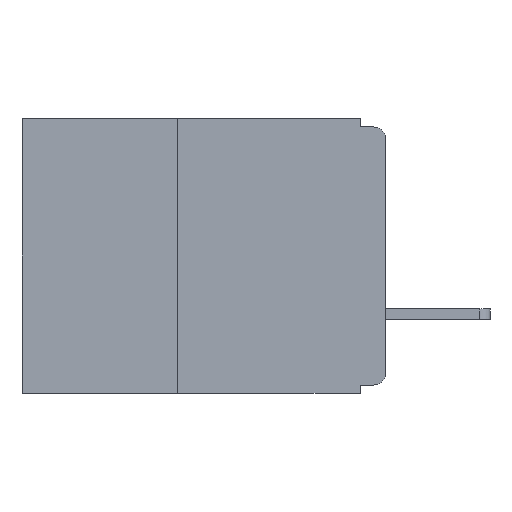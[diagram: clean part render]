
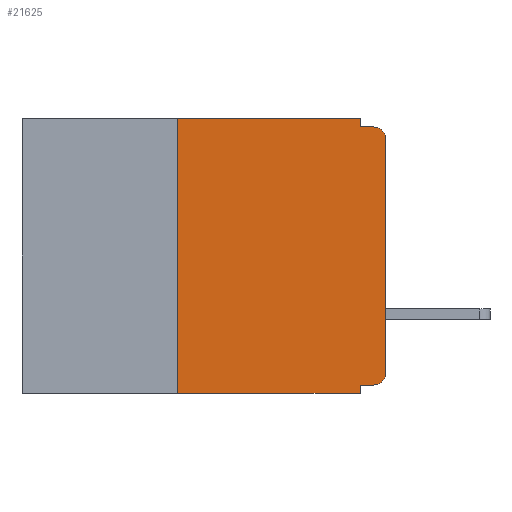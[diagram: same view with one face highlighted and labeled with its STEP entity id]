
A CAD part, left-side view. The second image highlights one B-rep face of the part: STEP entity #21625.
In plain terms, the highlighted planar face has unit normal (-1, 0, 0).
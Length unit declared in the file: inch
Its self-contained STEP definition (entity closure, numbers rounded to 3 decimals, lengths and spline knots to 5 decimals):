
#782 = DIRECTION ( 'NONE',  ( 0., -1., 0. ) ) ;
#1900 = ORIENTED_EDGE ( 'NONE', *, *, #23454, .F. ) ;
#1910 = VERTEX_POINT ( 'NONE', #27056 ) ;
#2072 = VECTOR ( 'NONE', #27822, 39.37008 ) ;
#3040 = CARTESIAN_POINT ( 'NONE',  ( 0., 0.031, -0.01 ) ) ;
#3853 = CARTESIAN_POINT ( 'NONE',  ( 0., 0.031, -0.33 ) ) ;
#4433 = VERTEX_POINT ( 'NONE', #3853 ) ;
#5592 = ORIENTED_EDGE ( 'NONE', *, *, #25178, .F. ) ;
#6671 = VERTEX_POINT ( 'NONE', #10846 ) ;
#6710 = EDGE_CURVE ( 'NONE', #1910, #20465, #29688, .T. ) ;
#7368 = LINE ( 'NONE', #30881, #26760 ) ;
#7585 = CARTESIAN_POINT ( 'NONE',  ( 0., 0.031, 0. ) ) ;
#7941 = CARTESIAN_POINT ( 'NONE',  ( 0., 0.25, -0.33 ) ) ;
#8379 = CIRCLE ( 'NONE', #24400, 0.015 ) ;
#8435 = ORIENTED_EDGE ( 'NONE', *, *, #30061, .T. ) ;
#8722 = VERTEX_POINT ( 'NONE', #14818 ) ;
#9685 = DIRECTION ( 'NONE',  ( 0., 0., -1. ) ) ;
#9710 = DIRECTION ( 'NONE',  ( -1., 0., 0. ) ) ;
#9717 = CARTESIAN_POINT ( 'NONE',  ( 0., 0.015, -0.025 ) ) ;
#9826 = DIRECTION ( 'NONE',  ( 0., 1., 0. ) ) ;
#9896 = AXIS2_PLACEMENT_3D ( 'NONE', #9717, #9710, #9685 ) ;
#10846 = CARTESIAN_POINT ( 'NONE',  ( 0., 0.031, 0. ) ) ;
#11538 = CARTESIAN_POINT ( 'NONE',  ( 0., 0.015, -0.305 ) ) ;
#11720 = VECTOR ( 'NONE', #9826, 39.37008 ) ;
#11738 = ORIENTED_EDGE ( 'NONE', *, *, #24427, .T. ) ;
#12065 = EDGE_CURVE ( 'NONE', #8722, #18976, #19317, .T. ) ;
#12128 = ORIENTED_EDGE ( 'NONE', *, *, #26253, .F. ) ;
#12326 = CARTESIAN_POINT ( 'NONE',  ( 0., 0.25, -0.33 ) ) ;
#13270 = FACE_OUTER_BOUND ( 'NONE', #25544, .T. ) ;
#13372 = DIRECTION ( 'NONE',  ( 1., 0., 0. ) ) ;
#13561 = DIRECTION ( 'NONE',  ( 0., -1., 0. ) ) ;
#13675 = VECTOR ( 'NONE', #21478, 39.37008 ) ;
#13900 = CARTESIAN_POINT ( 'NONE',  ( 0., 0.437, 0. ) ) ;
#14158 = DIRECTION ( 'NONE',  ( 0., 0., -1. ) ) ;
#14600 = ORIENTED_EDGE ( 'NONE', *, *, #25430, .F. ) ;
#14818 = CARTESIAN_POINT ( 'NONE',  ( 0., 0.015, -0.32 ) ) ;
#14859 = CARTESIAN_POINT ( 'NONE',  ( 0., 0., -0.32 ) ) ;
#15343 = CARTESIAN_POINT ( 'NONE',  ( 0., 0., -0.305 ) ) ;
#15831 = ORIENTED_EDGE ( 'NONE', *, *, #12065, .F. ) ;
#16250 = VECTOR ( 'NONE', #13561, 39.37008 ) ;
#16925 = ORIENTED_EDGE ( 'NONE', *, *, #6710, .T. ) ;
#17311 = VECTOR ( 'NONE', #32391, 39.37008 ) ;
#17807 = VERTEX_POINT ( 'NONE', #3040 ) ;
#18728 = VECTOR ( 'NONE', #27513, 39.37008 ) ;
#18751 = VERTEX_POINT ( 'NONE', #29865 ) ;
#18976 = VERTEX_POINT ( 'NONE', #26283 ) ;
#19317 = LINE ( 'NONE', #14859, #11720 ) ;
#20465 = VERTEX_POINT ( 'NONE', #27160 ) ;
#21439 = CARTESIAN_POINT ( 'NONE',  ( 0., 0., -0.01 ) ) ;
#21478 = DIRECTION ( 'NONE',  ( 0., -1., 0. ) ) ;
#21625 = ADVANCED_FACE ( 'NONE', ( #13270 ), #23345, .F. ) ;
#21923 = LINE ( 'NONE', #13900, #13675 ) ;
#22624 = EDGE_CURVE ( 'NONE', #6671, #17807, #29143, .T. ) ;
#23169 = ORIENTED_EDGE ( 'NONE', *, *, #22624, .F. ) ;
#23345 = PLANE ( 'NONE',  #32097 ) ;
#23454 = EDGE_CURVE ( 'NONE', #18976, #4433, #7368, .T. ) ;
#23763 = DIRECTION ( 'NONE',  ( 0., 0., -1. ) ) ;
#23917 = LINE ( 'NONE', #12326, #17311 ) ;
#24400 = AXIS2_PLACEMENT_3D ( 'NONE', #11538, #29065, #14158 ) ;
#24427 = EDGE_CURVE ( 'NONE', #26658, #4433, #29389, .T. ) ;
#24512 = LINE ( 'NONE', #25033, #18728 ) ;
#25033 = CARTESIAN_POINT ( 'NONE',  ( 0., 0., 0. ) ) ;
#25178 = EDGE_CURVE ( 'NONE', #17807, #20465, #25889, .T. ) ;
#25430 = EDGE_CURVE ( 'NONE', #26658, #18751, #23917, .T. ) ;
#25544 = EDGE_LOOP ( 'NONE', ( #8435, #16925, #5592, #23169, #12128, #14600, #11738, #1900, #15831, #32851 ) ) ;
#25889 = LINE ( 'NONE', #21439, #31648 ) ;
#26253 = EDGE_CURVE ( 'NONE', #18751, #6671, #21923, .T. ) ;
#26283 = CARTESIAN_POINT ( 'NONE',  ( 0., 0.031, -0.32 ) ) ;
#26658 = VERTEX_POINT ( 'NONE', #7941 ) ;
#26760 = VECTOR ( 'NONE', #23763, 39.37008 ) ;
#27056 = CARTESIAN_POINT ( 'NONE',  ( 0., 0., -0.025 ) ) ;
#27160 = CARTESIAN_POINT ( 'NONE',  ( 0., 0.015, -0.01 ) ) ;
#27513 = DIRECTION ( 'NONE',  ( 0., 0., 1. ) ) ;
#27822 = DIRECTION ( 'NONE',  ( 0., 0., -1. ) ) ;
#28317 = CARTESIAN_POINT ( 'NONE',  ( 0., 0.437, 0. ) ) ;
#28328 = EDGE_CURVE ( 'NONE', #8722, #32456, #8379, .T. ) ;
#29065 = DIRECTION ( 'NONE',  ( -1., 0., 0. ) ) ;
#29143 = LINE ( 'NONE', #7585, #2072 ) ;
#29389 = LINE ( 'NONE', #32319, #16250 ) ;
#29688 = CIRCLE ( 'NONE', #9896, 0.015 ) ;
#29865 = CARTESIAN_POINT ( 'NONE',  ( 0., 0.25, 0. ) ) ;
#30061 = EDGE_CURVE ( 'NONE', #32456, #1910, #24512, .T. ) ;
#30766 = DIRECTION ( 'NONE',  ( 0., 0., -1. ) ) ;
#30881 = CARTESIAN_POINT ( 'NONE',  ( 0., 0.031, -0.33 ) ) ;
#31648 = VECTOR ( 'NONE', #782, 39.37008 ) ;
#32097 = AXIS2_PLACEMENT_3D ( 'NONE', #28317, #13372, #30766 ) ;
#32319 = CARTESIAN_POINT ( 'NONE',  ( 0., 0.437, -0.33 ) ) ;
#32391 = DIRECTION ( 'NONE',  ( 0., 0., 1. ) ) ;
#32456 = VERTEX_POINT ( 'NONE', #15343 ) ;
#32851 = ORIENTED_EDGE ( 'NONE', *, *, #28328, .T. ) ;
